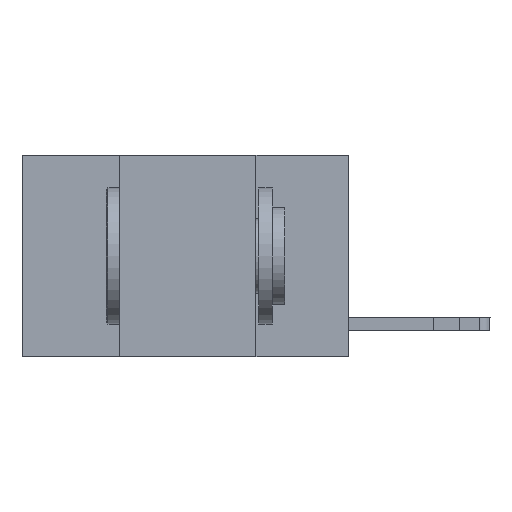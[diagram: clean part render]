
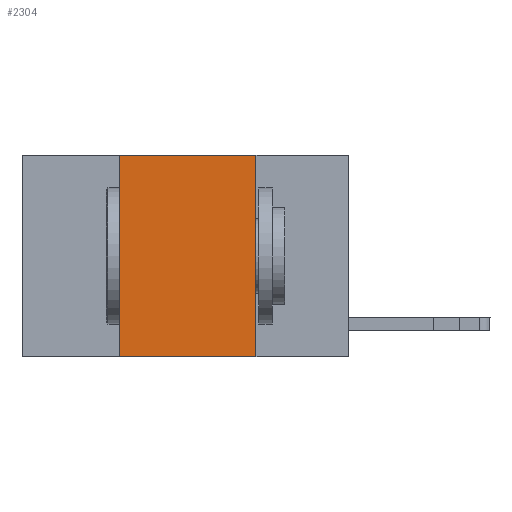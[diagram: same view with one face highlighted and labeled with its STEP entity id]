
A CAD part, left-side view. The second image highlights one B-rep face of the part: STEP entity #2304.
In plain terms, the highlighted planar face has unit normal (-1, 0, 0).
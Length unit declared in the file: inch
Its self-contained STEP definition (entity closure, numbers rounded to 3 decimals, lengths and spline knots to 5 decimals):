
#293 = VERTEX_POINT ( 'NONE', #10959 ) ;
#478 = CARTESIAN_POINT ( 'NONE',  ( 0., 0.42, 0. ) ) ;
#822 = PLANE ( 'NONE',  #24576 ) ;
#1881 = ORIENTED_EDGE ( 'NONE', *, *, #8458, .F. ) ;
#2102 = VECTOR ( 'NONE', #26716, 39.37008 ) ;
#2304 = ADVANCED_FACE ( 'NONE', ( #21197 ), #822, .F. ) ;
#3669 = VERTEX_POINT ( 'NONE', #6319 ) ;
#3952 = LINE ( 'NONE', #14259, #25025 ) ;
#4277 = DIRECTION ( 'NONE',  ( 1., 0., 0. ) ) ;
#6319 = CARTESIAN_POINT ( 'NONE',  ( 0., 0.17, -0.37 ) ) ;
#6660 = DIRECTION ( 'NONE',  ( 0., 0., 1. ) ) ;
#7450 = VERTEX_POINT ( 'NONE', #25584 ) ;
#8102 = DIRECTION ( 'NONE',  ( 0., -1., 0. ) ) ;
#8317 = VECTOR ( 'NONE', #6660, 39.37008 ) ;
#8458 = EDGE_CURVE ( 'NONE', #293, #3669, #15299, .T. ) ;
#8988 = LINE ( 'NONE', #19254, #8317 ) ;
#9793 = CARTESIAN_POINT ( 'NONE',  ( 0., 0.17, 0. ) ) ;
#10959 = CARTESIAN_POINT ( 'NONE',  ( 0., 0.17, 0. ) ) ;
#12048 = CARTESIAN_POINT ( 'NONE',  ( 0., 0.6, -0.37 ) ) ;
#12137 = VERTEX_POINT ( 'NONE', #478 ) ;
#13322 = LINE ( 'NONE', #12048, #2102 ) ;
#13752 = ORIENTED_EDGE ( 'NONE', *, *, #22023, .F. ) ;
#14259 = CARTESIAN_POINT ( 'NONE',  ( 0., 0.6, 0. ) ) ;
#15074 = ORIENTED_EDGE ( 'NONE', *, *, #25887, .F. ) ;
#15299 = LINE ( 'NONE', #9793, #23835 ) ;
#16866 = CARTESIAN_POINT ( 'NONE',  ( 0., 0.6, 0. ) ) ;
#18996 = DIRECTION ( 'NONE',  ( 0., 0., -1. ) ) ;
#19254 = CARTESIAN_POINT ( 'NONE',  ( 0., 0.42, 0. ) ) ;
#20636 = ORIENTED_EDGE ( 'NONE', *, *, #25042, .T. ) ;
#21197 = FACE_OUTER_BOUND ( 'NONE', #22361, .T. ) ;
#22023 = EDGE_CURVE ( 'NONE', #12137, #293, #3952, .T. ) ;
#22361 = EDGE_LOOP ( 'NONE', ( #1881, #13752, #15074, #20636 ) ) ;
#23835 = VECTOR ( 'NONE', #26608, 39.37008 ) ;
#24576 = AXIS2_PLACEMENT_3D ( 'NONE', #16866, #4277, #18996 ) ;
#25025 = VECTOR ( 'NONE', #8102, 39.37008 ) ;
#25042 = EDGE_CURVE ( 'NONE', #7450, #3669, #13322, .T. ) ;
#25584 = CARTESIAN_POINT ( 'NONE',  ( 0., 0.42, -0.37 ) ) ;
#25887 = EDGE_CURVE ( 'NONE', #7450, #12137, #8988, .T. ) ;
#26608 = DIRECTION ( 'NONE',  ( 0., 0., -1. ) ) ;
#26716 = DIRECTION ( 'NONE',  ( 0., -1., 0. ) ) ;
